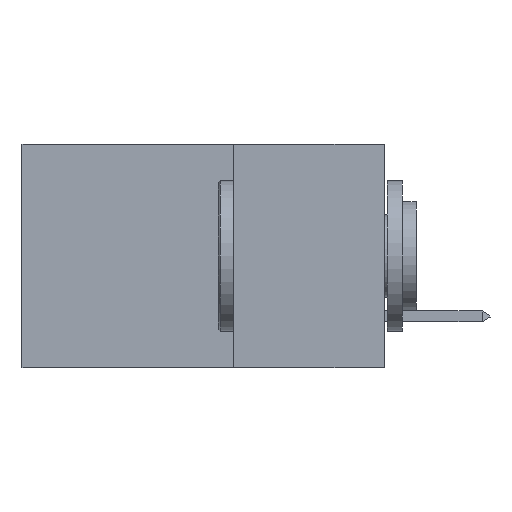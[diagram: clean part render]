
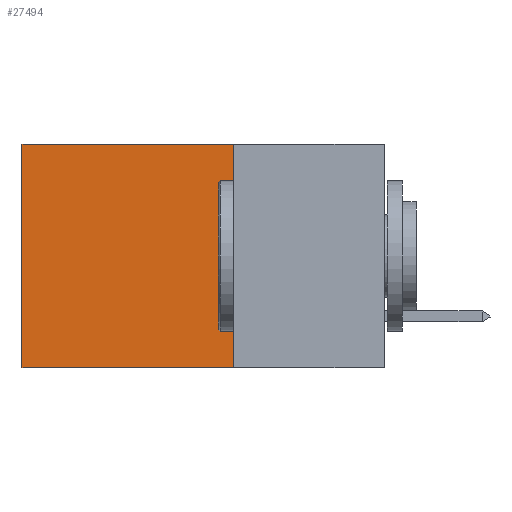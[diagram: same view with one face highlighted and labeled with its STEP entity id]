
A CAD part, left-side view. The second image highlights one B-rep face of the part: STEP entity #27494.
In plain terms, the highlighted planar face has unit normal (-1, 0, 0).
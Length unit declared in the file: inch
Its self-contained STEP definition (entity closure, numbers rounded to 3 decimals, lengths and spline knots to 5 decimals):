
#1315 = LINE ( 'NONE', #9933, #13834 ) ;
#1348 = VECTOR ( 'NONE', #8074, 39.37008 ) ;
#3160 = ORIENTED_EDGE ( 'NONE', *, *, #9483, .T. ) ;
#4266 = VERTEX_POINT ( 'NONE', #12446 ) ;
#5677 = ORIENTED_EDGE ( 'NONE', *, *, #13403, .F. ) ;
#5815 = DIRECTION ( 'NONE',  ( 0., 0., -1. ) ) ;
#7786 = LINE ( 'NONE', #27317, #1348 ) ;
#8074 = DIRECTION ( 'NONE',  ( 0., 1., 0. ) ) ;
#8812 = AXIS2_PLACEMENT_3D ( 'NONE', #16275, #11916, #11739 ) ;
#9278 = LINE ( 'NONE', #10093, #24527 ) ;
#9449 = CARTESIAN_POINT ( 'NONE',  ( 0.2875, 0.6, -0.37 ) ) ;
#9483 = EDGE_CURVE ( 'NONE', #20924, #16590, #1315, .T. ) ;
#9933 = CARTESIAN_POINT ( 'NONE',  ( 0.2875, 0.6, 0. ) ) ;
#10093 = CARTESIAN_POINT ( 'NONE',  ( 0.2875, 0.25, 0. ) ) ;
#10619 = CARTESIAN_POINT ( 'NONE',  ( 0.2875, 0.25, 0. ) ) ;
#11688 = VECTOR ( 'NONE', #25774, 39.37008 ) ;
#11739 = DIRECTION ( 'NONE',  ( 0., 0., -1. ) ) ;
#11916 = DIRECTION ( 'NONE',  ( 1., 0., 0. ) ) ;
#12446 = CARTESIAN_POINT ( 'NONE',  ( 0.2875, 0.25, 0. ) ) ;
#13403 = EDGE_CURVE ( 'NONE', #26919, #16590, #7786, .T. ) ;
#13834 = VECTOR ( 'NONE', #5815, 39.37008 ) ;
#16237 = EDGE_CURVE ( 'NONE', #4266, #26919, #17745, .T. ) ;
#16275 = CARTESIAN_POINT ( 'NONE',  ( 0.2875, 0.25, 0. ) ) ;
#16590 = VERTEX_POINT ( 'NONE', #9449 ) ;
#16800 = DIRECTION ( 'NONE',  ( 0., 1., 0. ) ) ;
#17745 = LINE ( 'NONE', #10619, #11688 ) ;
#17928 = CARTESIAN_POINT ( 'NONE',  ( 0.2875, 0.6, 0. ) ) ;
#20370 = FACE_OUTER_BOUND ( 'NONE', #26755, .T. ) ;
#20924 = VERTEX_POINT ( 'NONE', #17928 ) ;
#24287 = ORIENTED_EDGE ( 'NONE', *, *, #24738, .T. ) ;
#24527 = VECTOR ( 'NONE', #16800, 39.37008 ) ;
#24738 = EDGE_CURVE ( 'NONE', #4266, #20924, #9278, .T. ) ;
#25774 = DIRECTION ( 'NONE',  ( 0., 0., -1. ) ) ;
#26618 = ORIENTED_EDGE ( 'NONE', *, *, #16237, .F. ) ;
#26755 = EDGE_LOOP ( 'NONE', ( #3160, #5677, #26618, #24287 ) ) ;
#26767 = CARTESIAN_POINT ( 'NONE',  ( 0.2875, 0.25, -0.37 ) ) ;
#26919 = VERTEX_POINT ( 'NONE', #26767 ) ;
#27293 = PLANE ( 'NONE',  #8812 ) ;
#27317 = CARTESIAN_POINT ( 'NONE',  ( 0.2875, 0.25, -0.37 ) ) ;
#27494 = ADVANCED_FACE ( 'NONE', ( #20370 ), #27293, .F. ) ;
